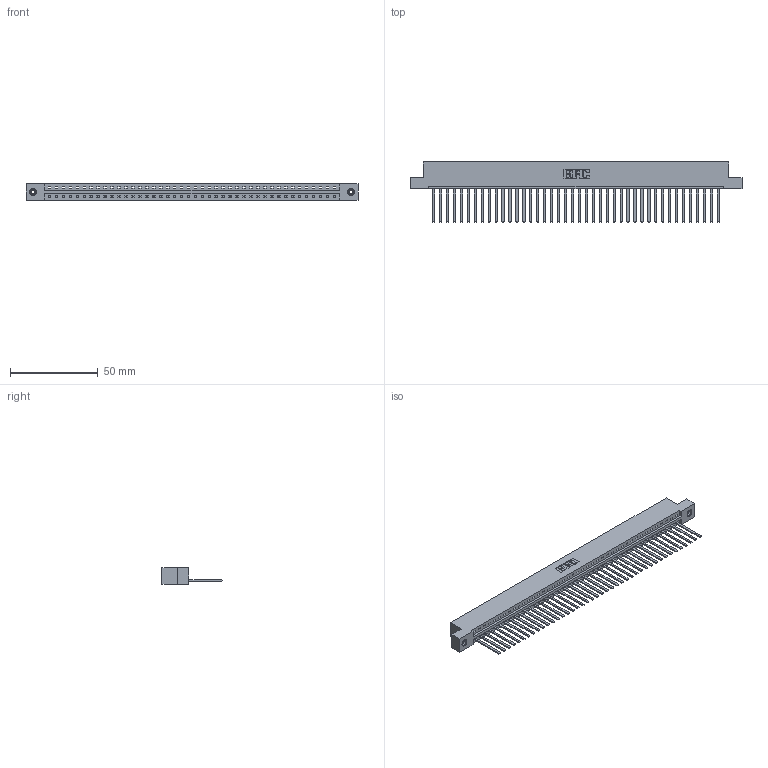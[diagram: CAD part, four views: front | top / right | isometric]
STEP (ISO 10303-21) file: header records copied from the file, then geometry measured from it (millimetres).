
FILE_DESCRIPTION (( 'STEP AP203' ), '1' );
FILE_NAME ('387-042-544-108.STEP', '2018-09-19T23:06:42', ( '' ), ( '' ), 'SwSTEP 2.0', 'SolidWorks 2016', '' );
FILE_SCHEMA (( 'CONFIG_CONTROL_DESIGN' ));
Length unit declared in the file: inch
Products named in the file (4): 337 Part_Flush Mounting Lugs - 0.156 Dia-TI; 345-292-001_345-293-144; 345-250-001_345-250-003-102; 387-042-544-108
Assembly tree (45 placements, depth 2):
  387-042-544-108
    337 Part_Flush Mounting Lugs - 0.156 Dia-TI
    345-292-001_345-293-144  x42
    345-250-001_345-250-003-102  x2
Bounding box: 189.43 x 34.3 x 9.4 mm (x, y, z)
Volume: 20168.3 mm3; surface area: 22470.8 mm2
Topology: 45 solids, 45 shells, 2526 faces, 7587 edges, 4994 vertices
Faces by surface type: plane 1866, cylinder 644, cone 12, torus 4
Entity records: 32222 total; most frequent: CARTESIAN_POINT 5591, ORIENTED_EDGE 5562, DIRECTION 4735, EDGE_CURVE 2781, LINE 2637, VECTOR 2637, VERTEX_POINT 1848, AXIS2_PLACEMENT_3D 1049
